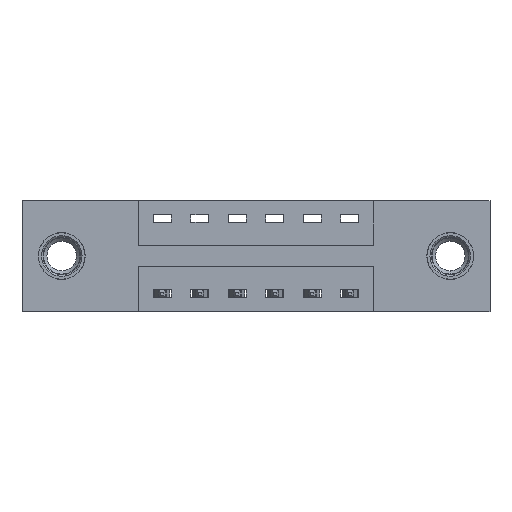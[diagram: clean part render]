
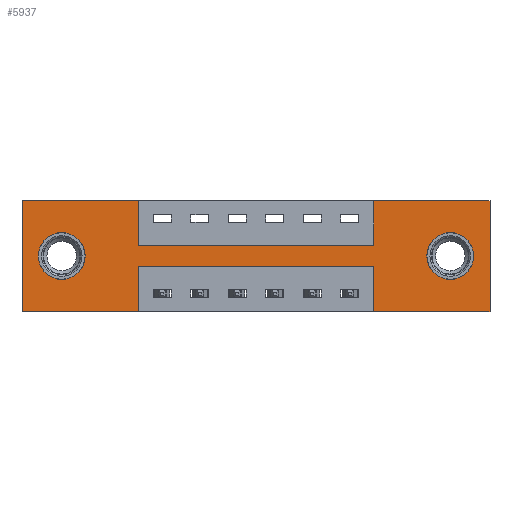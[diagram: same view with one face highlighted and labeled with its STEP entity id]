
A CAD part, front view. The second image highlights one B-rep face of the part: STEP entity #5937.
In plain terms, the highlighted planar face has unit normal (0, -1, 0).
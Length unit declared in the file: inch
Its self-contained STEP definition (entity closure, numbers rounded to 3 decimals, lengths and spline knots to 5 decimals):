
#13 = CARTESIAN_POINT ( 'NONE',  ( 1.1725, 0., -0.37 ) ) ;
#27 = AXIS2_PLACEMENT_3D ( 'NONE', #8565, #4048, #9298 ) ;
#78 = VERTEX_POINT ( 'NONE', #1391 ) ;
#87 = DIRECTION ( 'NONE',  ( -1., 0., 0. ) ) ;
#216 = VERTEX_POINT ( 'NONE', #4583 ) ;
#224 = DIRECTION ( 'NONE',  ( 0., 0., -1. ) ) ;
#392 = EDGE_CURVE ( 'NONE', #78, #8674, #7342, .T. ) ;
#396 = LINE ( 'NONE', #1663, #3738 ) ;
#422 = EDGE_CURVE ( 'NONE', #6429, #7247, #9557, .T. ) ;
#699 = DIRECTION ( 'NONE',  ( 0., 1., 0. ) ) ;
#980 = EDGE_CURVE ( 'NONE', #9309, #9183, #4388, .T. ) ;
#988 = VERTEX_POINT ( 'NONE', #8527 ) ;
#1047 = CIRCLE ( 'NONE', #6121, 0.078 ) ;
#1334 = ORIENTED_EDGE ( 'NONE', *, *, #5198, .F. ) ;
#1374 = EDGE_LOOP ( 'NONE', ( #6199, #8449 ) ) ;
#1391 = CARTESIAN_POINT ( 'NONE',  ( 1.56, 0., 0. ) ) ;
#1392 = CARTESIAN_POINT ( 'NONE',  ( 1.1725, 0., 0. ) ) ;
#1643 = CARTESIAN_POINT ( 'NONE',  ( 0., 0., -0.37 ) ) ;
#1663 = CARTESIAN_POINT ( 'NONE',  ( 0., 0., 0. ) ) ;
#1734 = VERTEX_POINT ( 'NONE', #2106 ) ;
#1851 = CIRCLE ( 'NONE', #5210, 0.078 ) ;
#1878 = DIRECTION ( 'NONE',  ( 0., 0., 1. ) ) ;
#1969 = VECTOR ( 'NONE', #7443, 39.37008 ) ;
#2106 = CARTESIAN_POINT ( 'NONE',  ( 1.1725, 0., -0.22 ) ) ;
#2408 = VERTEX_POINT ( 'NONE', #7661 ) ;
#2483 = CARTESIAN_POINT ( 'NONE',  ( 0., 0., -0.37 ) ) ;
#2758 = LINE ( 'NONE', #4247, #8762 ) ;
#2780 = VERTEX_POINT ( 'NONE', #5933 ) ;
#2787 = VERTEX_POINT ( 'NONE', #1392 ) ;
#2914 = FACE_OUTER_BOUND ( 'NONE', #5188, .T. ) ;
#2947 = CARTESIAN_POINT ( 'NONE',  ( 1.1725, 0., -0.37 ) ) ;
#2999 = CARTESIAN_POINT ( 'NONE',  ( 0.3875, 0., 0. ) ) ;
#3072 = DIRECTION ( 'NONE',  ( 0., 0., -1. ) ) ;
#3149 = ORIENTED_EDGE ( 'NONE', *, *, #3933, .F. ) ;
#3268 = CARTESIAN_POINT ( 'NONE',  ( 1.56, 0., 0. ) ) ;
#3434 = CARTESIAN_POINT ( 'NONE',  ( 0.1325, 0., -0.185 ) ) ;
#3540 = VERTEX_POINT ( 'NONE', #2999 ) ;
#3563 = EDGE_CURVE ( 'NONE', #1734, #7589, #8235, .T. ) ;
#3612 = ORIENTED_EDGE ( 'NONE', *, *, #392, .F. ) ;
#3640 = DIRECTION ( 'NONE',  ( 1., 0., 0. ) ) ;
#3738 = VECTOR ( 'NONE', #9195, 39.37008 ) ;
#3757 = DIRECTION ( 'NONE',  ( -1., 0., 0. ) ) ;
#3802 = DIRECTION ( 'NONE',  ( 0., 0., -1. ) ) ;
#3807 = EDGE_CURVE ( 'NONE', #7247, #6429, #1851, .T. ) ;
#3852 = ORIENTED_EDGE ( 'NONE', *, *, #6851, .F. ) ;
#3871 = LINE ( 'NONE', #1643, #5864 ) ;
#3933 = EDGE_CURVE ( 'NONE', #7589, #9309, #5535, .T. ) ;
#3977 = CIRCLE ( 'NONE', #6704, 0.078 ) ;
#4048 = DIRECTION ( 'NONE',  ( 0., 1., 0. ) ) ;
#4135 = CARTESIAN_POINT ( 'NONE',  ( 0., 0., 0. ) ) ;
#4175 = DIRECTION ( 'NONE',  ( 0., 0., 1. ) ) ;
#4200 = DIRECTION ( 'NONE',  ( 0., 1., 0. ) ) ;
#4247 = CARTESIAN_POINT ( 'NONE',  ( 0.3875, 0., -0.15 ) ) ;
#4317 = ORIENTED_EDGE ( 'NONE', *, *, #8618, .F. ) ;
#4367 = CARTESIAN_POINT ( 'NONE',  ( 0.3875, 0., -0.37 ) ) ;
#4377 = CARTESIAN_POINT ( 'NONE',  ( 0.3875, 0., -0.22 ) ) ;
#4388 = LINE ( 'NONE', #2483, #4636 ) ;
#4556 = ORIENTED_EDGE ( 'NONE', *, *, #9545, .F. ) ;
#4583 = CARTESIAN_POINT ( 'NONE',  ( 0., 0., 0. ) ) ;
#4636 = VECTOR ( 'NONE', #6999, 39.37008 ) ;
#4675 = ORIENTED_EDGE ( 'NONE', *, *, #5584, .T. ) ;
#4912 = FACE_BOUND ( 'NONE', #9660, .T. ) ;
#5188 = EDGE_LOOP ( 'NONE', ( #3149, #9133, #1334, #9363, #3612, #7622, #3852, #5847, #4317, #6317, #4556, #6794 ) ) ;
#5198 = EDGE_CURVE ( 'NONE', #5961, #1734, #7522, .T. ) ;
#5210 = AXIS2_PLACEMENT_3D ( 'NONE', #8720, #4200, #9458 ) ;
#5232 = CARTESIAN_POINT ( 'NONE',  ( 0., 0., -0.37 ) ) ;
#5246 = CARTESIAN_POINT ( 'NONE',  ( 0.1325, 0., -0.185 ) ) ;
#5281 = CARTESIAN_POINT ( 'NONE',  ( 0.3875, 0., 0. ) ) ;
#5295 = CARTESIAN_POINT ( 'NONE',  ( 0., 0., -0.37 ) ) ;
#5345 = VECTOR ( 'NONE', #224, 39.37008 ) ;
#5360 = EDGE_CURVE ( 'NONE', #8674, #5961, #3871, .T. ) ;
#5535 = LINE ( 'NONE', #4367, #9295 ) ;
#5584 = EDGE_CURVE ( 'NONE', #2780, #8255, #3977, .T. ) ;
#5652 = DIRECTION ( 'NONE',  ( 0., 0., 1. ) ) ;
#5801 = LINE ( 'NONE', #7388, #9546 ) ;
#5847 = ORIENTED_EDGE ( 'NONE', *, *, #7478, .F. ) ;
#5864 = VECTOR ( 'NONE', #87, 39.37008 ) ;
#5933 = CARTESIAN_POINT ( 'NONE',  ( 0.1325, 0., -0.107 ) ) ;
#5937 = ADVANCED_FACE ( 'NONE', ( #6914, #4912, #2914 ), #6813, .T. ) ;
#5961 = VERTEX_POINT ( 'NONE', #13 ) ;
#5990 = VECTOR ( 'NONE', #3757, 39.37008 ) ;
#6013 = DIRECTION ( 'NONE',  ( 0., 0., 1. ) ) ;
#6068 = EDGE_CURVE ( 'NONE', #216, #3540, #396, .T. ) ;
#6121 = AXIS2_PLACEMENT_3D ( 'NONE', #5246, #699, #6013 ) ;
#6158 = CARTESIAN_POINT ( 'NONE',  ( 0.3875, 0., -0.37 ) ) ;
#6199 = ORIENTED_EDGE ( 'NONE', *, *, #3807, .T. ) ;
#6317 = ORIENTED_EDGE ( 'NONE', *, *, #6068, .F. ) ;
#6392 = CARTESIAN_POINT ( 'NONE',  ( 1.1725, 0., 0. ) ) ;
#6429 = VERTEX_POINT ( 'NONE', #6663 ) ;
#6498 = LINE ( 'NONE', #4135, #8282 ) ;
#6517 = VECTOR ( 'NONE', #3802, 39.37008 ) ;
#6620 = LINE ( 'NONE', #5281, #6517 ) ;
#6657 = VECTOR ( 'NONE', #1878, 39.37008 ) ;
#6663 = CARTESIAN_POINT ( 'NONE',  ( 1.4275, 0., -0.263 ) ) ;
#6667 = ORIENTED_EDGE ( 'NONE', *, *, #8563, .T. ) ;
#6704 = AXIS2_PLACEMENT_3D ( 'NONE', #3434, #8694, #4175 ) ;
#6794 = ORIENTED_EDGE ( 'NONE', *, *, #980, .F. ) ;
#6813 = PLANE ( 'NONE',  #8542 ) ;
#6851 = EDGE_CURVE ( 'NONE', #988, #2787, #8437, .T. ) ;
#6862 = CARTESIAN_POINT ( 'NONE',  ( 1.56, 0., -0.37 ) ) ;
#6914 = FACE_BOUND ( 'NONE', #1374, .T. ) ;
#6999 = DIRECTION ( 'NONE',  ( -1., 0., 0. ) ) ;
#7247 = VERTEX_POINT ( 'NONE', #8476 ) ;
#7342 = LINE ( 'NONE', #3268, #5345 ) ;
#7388 = CARTESIAN_POINT ( 'NONE',  ( 0., 0., 0. ) ) ;
#7443 = DIRECTION ( 'NONE',  ( 0., 0., 1. ) ) ;
#7478 = EDGE_CURVE ( 'NONE', #2408, #988, #2758, .T. ) ;
#7522 = LINE ( 'NONE', #2947, #1969 ) ;
#7569 = DIRECTION ( 'NONE',  ( 0., -1., 0. ) ) ;
#7589 = VERTEX_POINT ( 'NONE', #4377 ) ;
#7622 = ORIENTED_EDGE ( 'NONE', *, *, #8485, .F. ) ;
#7661 = CARTESIAN_POINT ( 'NONE',  ( 0.3875, 0., -0.15 ) ) ;
#8235 = LINE ( 'NONE', #9748, #5990 ) ;
#8255 = VERTEX_POINT ( 'NONE', #8582 ) ;
#8282 = VECTOR ( 'NONE', #5652, 39.37008 ) ;
#8437 = LINE ( 'NONE', #6392, #6657 ) ;
#8449 = ORIENTED_EDGE ( 'NONE', *, *, #422, .T. ) ;
#8476 = CARTESIAN_POINT ( 'NONE',  ( 1.4275, 0., -0.107 ) ) ;
#8485 = EDGE_CURVE ( 'NONE', #2787, #78, #5801, .T. ) ;
#8527 = CARTESIAN_POINT ( 'NONE',  ( 1.1725, 0., -0.15 ) ) ;
#8542 = AXIS2_PLACEMENT_3D ( 'NONE', #5295, #7569, #3072 ) ;
#8563 = EDGE_CURVE ( 'NONE', #8255, #2780, #1047, .T. ) ;
#8565 = CARTESIAN_POINT ( 'NONE',  ( 1.4275, 0., -0.185 ) ) ;
#8582 = CARTESIAN_POINT ( 'NONE',  ( 0.1325, 0., -0.263 ) ) ;
#8618 = EDGE_CURVE ( 'NONE', #3540, #2408, #6620, .T. ) ;
#8674 = VERTEX_POINT ( 'NONE', #6862 ) ;
#8694 = DIRECTION ( 'NONE',  ( 0., 1., 0. ) ) ;
#8720 = CARTESIAN_POINT ( 'NONE',  ( 1.4275, 0., -0.185 ) ) ;
#8762 = VECTOR ( 'NONE', #9498, 39.37008 ) ;
#8881 = DIRECTION ( 'NONE',  ( 0., 0., -1. ) ) ;
#9133 = ORIENTED_EDGE ( 'NONE', *, *, #3563, .F. ) ;
#9183 = VERTEX_POINT ( 'NONE', #5232 ) ;
#9195 = DIRECTION ( 'NONE',  ( 1., 0., 0. ) ) ;
#9295 = VECTOR ( 'NONE', #8881, 39.37008 ) ;
#9298 = DIRECTION ( 'NONE',  ( 0., 0., -1. ) ) ;
#9309 = VERTEX_POINT ( 'NONE', #6158 ) ;
#9363 = ORIENTED_EDGE ( 'NONE', *, *, #5360, .F. ) ;
#9458 = DIRECTION ( 'NONE',  ( 0., 0., -1. ) ) ;
#9498 = DIRECTION ( 'NONE',  ( 1., 0., 0. ) ) ;
#9545 = EDGE_CURVE ( 'NONE', #9183, #216, #6498, .T. ) ;
#9546 = VECTOR ( 'NONE', #3640, 39.37008 ) ;
#9557 = CIRCLE ( 'NONE', #27, 0.078 ) ;
#9660 = EDGE_LOOP ( 'NONE', ( #4675, #6667 ) ) ;
#9748 = CARTESIAN_POINT ( 'NONE',  ( 0.3875, 0., -0.22 ) ) ;
